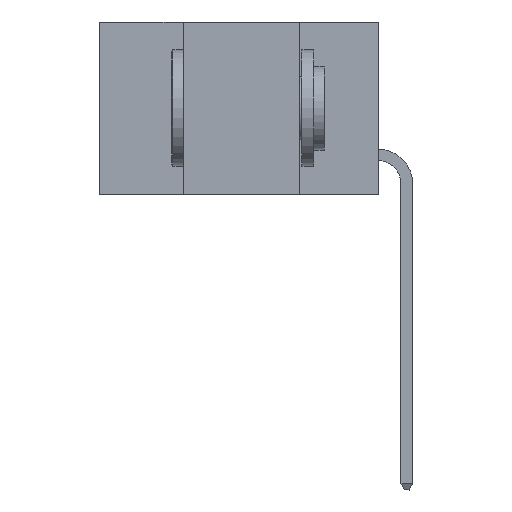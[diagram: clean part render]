
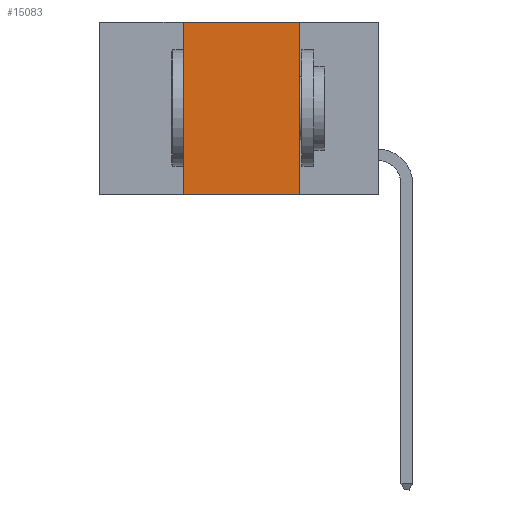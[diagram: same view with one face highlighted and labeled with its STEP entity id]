
A CAD part, left-side view. The second image highlights one B-rep face of the part: STEP entity #15083.
In plain terms, the highlighted planar face has unit normal (-1, 0, 0).
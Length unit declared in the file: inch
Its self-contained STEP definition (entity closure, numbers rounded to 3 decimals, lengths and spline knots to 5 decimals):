
#300 = EDGE_CURVE ( 'NONE', #8589, #9589, #7549, .T. ) ;
#506 = CARTESIAN_POINT ( 'NONE',  ( 0., 0.17, 0. ) ) ;
#510 = LINE ( 'NONE', #2335, #11192 ) ;
#696 = DIRECTION ( 'NONE',  ( 1., 0., 0. ) ) ;
#1208 = CARTESIAN_POINT ( 'NONE',  ( 0., 0.17, -0.37 ) ) ;
#1383 = LINE ( 'NONE', #12705, #5567 ) ;
#1619 = CARTESIAN_POINT ( 'NONE',  ( 0., 0.42, 0. ) ) ;
#1857 = ORIENTED_EDGE ( 'NONE', *, *, #6923, .F. ) ;
#2307 = CARTESIAN_POINT ( 'NONE',  ( 0., 0.42, -0.37 ) ) ;
#2335 = CARTESIAN_POINT ( 'NONE',  ( 0., 0.42, -0.37 ) ) ;
#2572 = CARTESIAN_POINT ( 'NONE',  ( 0., 0.6, -0.37 ) ) ;
#2682 = VERTEX_POINT ( 'NONE', #1619 ) ;
#2872 = VECTOR ( 'NONE', #14207, 39.37008 ) ;
#4803 = DIRECTION ( 'NONE',  ( 0., 0., -1. ) ) ;
#5080 = ORIENTED_EDGE ( 'NONE', *, *, #16262, .T. ) ;
#5567 = VECTOR ( 'NONE', #12858, 39.37008 ) ;
#5854 = EDGE_LOOP ( 'NONE', ( #9894, #11899, #1857, #5080 ) ) ;
#5892 = DIRECTION ( 'NONE',  ( 0., 0., -1. ) ) ;
#6923 = EDGE_CURVE ( 'NONE', #14793, #2682, #510, .T. ) ;
#7549 = LINE ( 'NONE', #12429, #9161 ) ;
#8589 = VERTEX_POINT ( 'NONE', #506 ) ;
#9154 = LINE ( 'NONE', #2572, #2872 ) ;
#9161 = VECTOR ( 'NONE', #4803, 39.37008 ) ;
#9589 = VERTEX_POINT ( 'NONE', #1208 ) ;
#9792 = PLANE ( 'NONE',  #13463 ) ;
#9894 = ORIENTED_EDGE ( 'NONE', *, *, #300, .F. ) ;
#11192 = VECTOR ( 'NONE', #11388, 39.37008 ) ;
#11388 = DIRECTION ( 'NONE',  ( 0., 0., 1. ) ) ;
#11899 = ORIENTED_EDGE ( 'NONE', *, *, #14843, .F. ) ;
#12096 = CARTESIAN_POINT ( 'NONE',  ( 0., 0.6, 0. ) ) ;
#12429 = CARTESIAN_POINT ( 'NONE',  ( 0., 0.17, -0.37 ) ) ;
#12705 = CARTESIAN_POINT ( 'NONE',  ( 0., 0.6, 0. ) ) ;
#12858 = DIRECTION ( 'NONE',  ( 0., -1., 0. ) ) ;
#13463 = AXIS2_PLACEMENT_3D ( 'NONE', #12096, #696, #5892 ) ;
#14207 = DIRECTION ( 'NONE',  ( 0., -1., 0. ) ) ;
#14674 = FACE_OUTER_BOUND ( 'NONE', #5854, .T. ) ;
#14793 = VERTEX_POINT ( 'NONE', #2307 ) ;
#14843 = EDGE_CURVE ( 'NONE', #2682, #8589, #1383, .T. ) ;
#15083 = ADVANCED_FACE ( 'NONE', ( #14674 ), #9792, .F. ) ;
#16262 = EDGE_CURVE ( 'NONE', #14793, #9589, #9154, .T. ) ;
